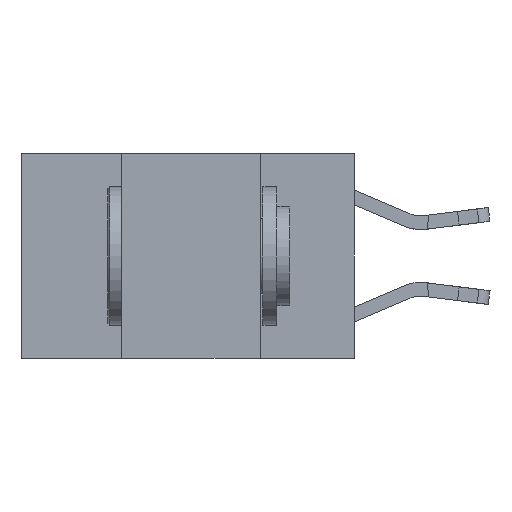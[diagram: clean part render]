
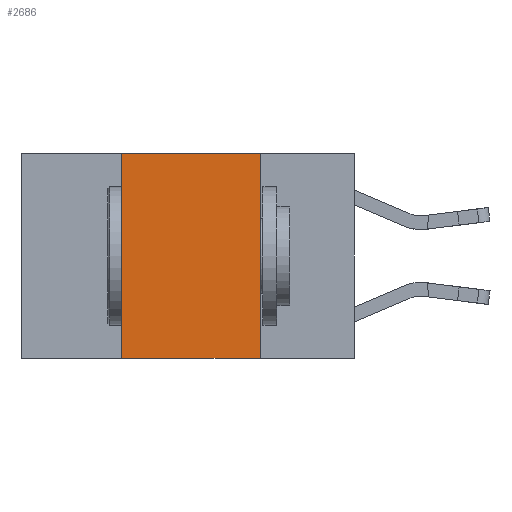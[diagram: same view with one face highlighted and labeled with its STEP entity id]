
A CAD part, left-side view. The second image highlights one B-rep face of the part: STEP entity #2686.
In plain terms, the highlighted planar face has unit normal (-1, 0, 0).
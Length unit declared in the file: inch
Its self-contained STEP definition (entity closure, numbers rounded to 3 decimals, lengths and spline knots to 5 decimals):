
#471 = CARTESIAN_POINT ( 'NONE',  ( 0., 0.17, 0. ) ) ;
#1345 = VERTEX_POINT ( 'NONE', #471 ) ;
#2150 = FACE_OUTER_BOUND ( 'NONE', #7235, .T. ) ;
#2686 = ADVANCED_FACE ( 'NONE', ( #2150 ), #16009, .F. ) ;
#3228 = CARTESIAN_POINT ( 'NONE',  ( 0., 0.42, 0. ) ) ;
#3603 = ORIENTED_EDGE ( 'NONE', *, *, #17472, .F. ) ;
#3619 = CARTESIAN_POINT ( 'NONE',  ( 0., 0.6, 0. ) ) ;
#3885 = VERTEX_POINT ( 'NONE', #9931 ) ;
#4066 = ORIENTED_EDGE ( 'NONE', *, *, #17814, .F. ) ;
#4745 = DIRECTION ( 'NONE',  ( 0., 0., 1. ) ) ;
#5151 = DIRECTION ( 'NONE',  ( 0., -1., 0. ) ) ;
#5360 = DIRECTION ( 'NONE',  ( 0., -1., 0. ) ) ;
#5389 = CARTESIAN_POINT ( 'NONE',  ( 0., 0.17, 0. ) ) ;
#5814 = LINE ( 'NONE', #5389, #13421 ) ;
#6313 = EDGE_CURVE ( 'NONE', #7656, #1345, #16123, .T. ) ;
#6980 = CARTESIAN_POINT ( 'NONE',  ( 0., 0.6, 0. ) ) ;
#7235 = EDGE_LOOP ( 'NONE', ( #3603, #19695, #4066, #12669 ) ) ;
#7656 = VERTEX_POINT ( 'NONE', #18240 ) ;
#7696 = LINE ( 'NONE', #3228, #15254 ) ;
#7923 = LINE ( 'NONE', #14413, #12459 ) ;
#8523 = DIRECTION ( 'NONE',  ( 0., 0., -1. ) ) ;
#8621 = VECTOR ( 'NONE', #5151, 39.37008 ) ;
#9739 = AXIS2_PLACEMENT_3D ( 'NONE', #6980, #17559, #8523 ) ;
#9931 = CARTESIAN_POINT ( 'NONE',  ( 0., 0.17, -0.37 ) ) ;
#9966 = DIRECTION ( 'NONE',  ( 0., 0., -1. ) ) ;
#9983 = CARTESIAN_POINT ( 'NONE',  ( 0., 0.42, -0.37 ) ) ;
#12459 = VECTOR ( 'NONE', #5360, 39.37008 ) ;
#12669 = ORIENTED_EDGE ( 'NONE', *, *, #17997, .T. ) ;
#13421 = VECTOR ( 'NONE', #9966, 39.37008 ) ;
#14413 = CARTESIAN_POINT ( 'NONE',  ( 0., 0.6, -0.37 ) ) ;
#15254 = VECTOR ( 'NONE', #4745, 39.37008 ) ;
#16009 = PLANE ( 'NONE',  #9739 ) ;
#16123 = LINE ( 'NONE', #3619, #8621 ) ;
#16992 = VERTEX_POINT ( 'NONE', #9983 ) ;
#17472 = EDGE_CURVE ( 'NONE', #1345, #3885, #5814, .T. ) ;
#17559 = DIRECTION ( 'NONE',  ( 1., 0., 0. ) ) ;
#17814 = EDGE_CURVE ( 'NONE', #16992, #7656, #7696, .T. ) ;
#17997 = EDGE_CURVE ( 'NONE', #16992, #3885, #7923, .T. ) ;
#18240 = CARTESIAN_POINT ( 'NONE',  ( 0., 0.42, 0. ) ) ;
#19695 = ORIENTED_EDGE ( 'NONE', *, *, #6313, .F. ) ;
